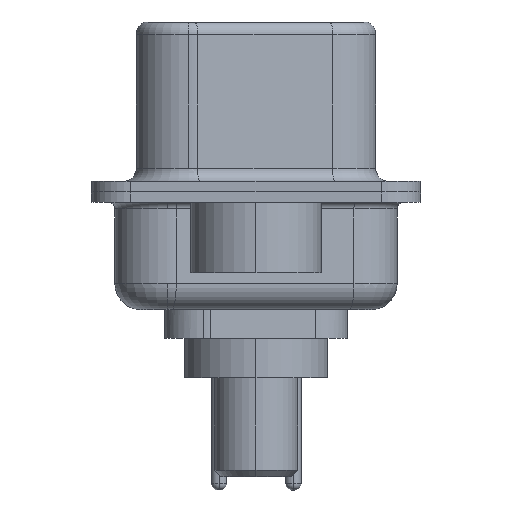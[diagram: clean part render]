
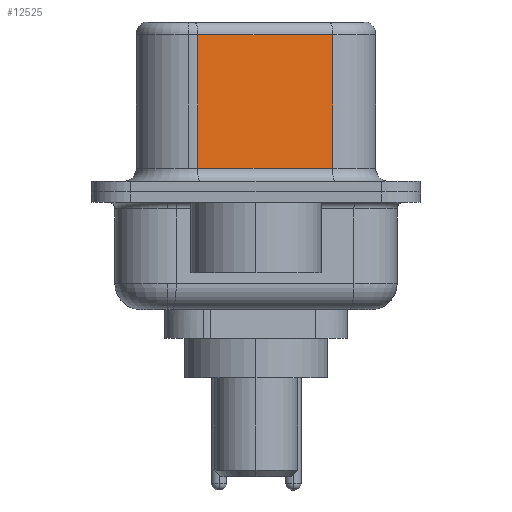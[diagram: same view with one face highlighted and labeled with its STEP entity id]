
A CAD part, left-side view. The second image highlights one B-rep face of the part: STEP entity #12525.
In plain terms, the highlighted planar face has unit normal (-0.985, -0.174, 0).
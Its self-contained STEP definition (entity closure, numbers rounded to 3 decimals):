
#386 = LINE ( 'NONE', #9534, #20425 ) ;
#874 = CARTESIAN_POINT ( 'NONE',  ( 4.585, -2.927, 0.9 ) ) ;
#934 = FACE_OUTER_BOUND ( 'NONE', #6554, .T. ) ;
#1405 = VECTOR ( 'NONE', #7992, 1000. ) ;
#1642 = CARTESIAN_POINT ( 'NONE',  ( 3.675, 2.233, 6.52 ) ) ;
#2538 = CARTESIAN_POINT ( 'NONE',  ( 4.585, -2.927, 6.52 ) ) ;
#2969 = EDGE_CURVE ( 'NONE', #3703, #14624, #12501, .T. ) ;
#3391 = VERTEX_POINT ( 'NONE', #874 ) ;
#3703 = VERTEX_POINT ( 'NONE', #11883 ) ;
#4616 = DIRECTION ( 'NONE',  ( 0.174, -0.985, 0. ) ) ;
#5589 = LINE ( 'NONE', #7752, #18070 ) ;
#5675 = LINE ( 'NONE', #2538, #1405 ) ;
#5728 = EDGE_CURVE ( 'NONE', #10957, #3391, #5675, .T. ) ;
#5966 = ORIENTED_EDGE ( 'NONE', *, *, #8041, .T. ) ;
#6554 = EDGE_LOOP ( 'NONE', ( #6950, #5966, #13642, #12351 ) ) ;
#6950 = ORIENTED_EDGE ( 'NONE', *, *, #5728, .F. ) ;
#7621 = CARTESIAN_POINT ( 'NONE',  ( 4.585, -2.927, 6.52 ) ) ;
#7752 = CARTESIAN_POINT ( 'NONE',  ( 4.585, -2.927, 6.02 ) ) ;
#7992 = DIRECTION ( 'NONE',  ( 0., 0., -1. ) ) ;
#8041 = EDGE_CURVE ( 'NONE', #10957, #3703, #5589, .T. ) ;
#8664 = CARTESIAN_POINT ( 'NONE',  ( 3.675, 2.233, 0.9 ) ) ;
#8696 = AXIS2_PLACEMENT_3D ( 'NONE', #7621, #9256, #20653 ) ;
#9256 = DIRECTION ( 'NONE',  ( 0.985, 0.174, 0. ) ) ;
#9534 = CARTESIAN_POINT ( 'NONE',  ( 4.585, -2.927, 0.9 ) ) ;
#10957 = VERTEX_POINT ( 'NONE', #16254 ) ;
#11883 = CARTESIAN_POINT ( 'NONE',  ( 3.675, 2.233, 6.02 ) ) ;
#12351 = ORIENTED_EDGE ( 'NONE', *, *, #13762, .T. ) ;
#12501 = LINE ( 'NONE', #1642, #16763 ) ;
#12525 = ADVANCED_FACE ( 'NONE', ( #934 ), #17392, .F. ) ;
#13642 = ORIENTED_EDGE ( 'NONE', *, *, #2969, .T. ) ;
#13762 = EDGE_CURVE ( 'NONE', #14624, #3391, #386, .T. ) ;
#14326 = DIRECTION ( 'NONE',  ( 0., 0., -1. ) ) ;
#14624 = VERTEX_POINT ( 'NONE', #8664 ) ;
#16254 = CARTESIAN_POINT ( 'NONE',  ( 4.585, -2.927, 6.02 ) ) ;
#16763 = VECTOR ( 'NONE', #14326, 1000. ) ;
#17392 = PLANE ( 'NONE',  #8696 ) ;
#18070 = VECTOR ( 'NONE', #19788, 1000. ) ;
#19788 = DIRECTION ( 'NONE',  ( -0.174, 0.985, 0. ) ) ;
#20425 = VECTOR ( 'NONE', #4616, 1000. ) ;
#20653 = DIRECTION ( 'NONE',  ( -0.174, 0.985, 0. ) ) ;
